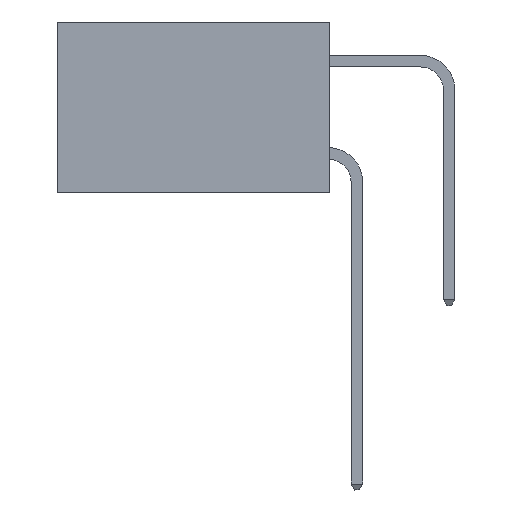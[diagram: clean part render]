
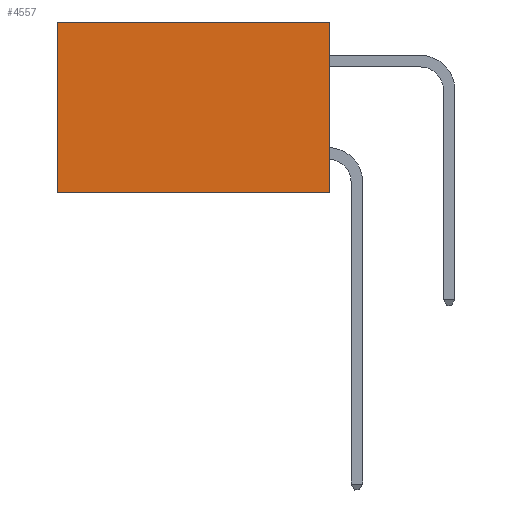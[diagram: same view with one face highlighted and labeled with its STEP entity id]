
A CAD part, left-side view. The second image highlights one B-rep face of the part: STEP entity #4557.
In plain terms, the highlighted planar face has unit normal (-1, 0, 0).
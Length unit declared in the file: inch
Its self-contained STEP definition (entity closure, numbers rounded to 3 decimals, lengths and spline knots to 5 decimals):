
#409 = VECTOR ( 'NONE', #18096, 39.37008 ) ;
#3427 = LINE ( 'NONE', #28919, #17047 ) ;
#3834 = VERTEX_POINT ( 'NONE', #17216 ) ;
#4557 = ADVANCED_FACE ( 'NONE', ( #15839 ), #34240, .F. ) ;
#5149 = ORIENTED_EDGE ( 'NONE', *, *, #21586, .T. ) ;
#5661 = VECTOR ( 'NONE', #33247, 39.37008 ) ;
#6301 = AXIS2_PLACEMENT_3D ( 'NONE', #33501, #33183, #33338 ) ;
#6411 = CARTESIAN_POINT ( 'NONE',  ( 0.277, 0., -0.37 ) ) ;
#6700 = ORIENTED_EDGE ( 'NONE', *, *, #19573, .T. ) ;
#6984 = VERTEX_POINT ( 'NONE', #6411 ) ;
#9887 = DIRECTION ( 'NONE',  ( 0., 1., 0. ) ) ;
#12325 = LINE ( 'NONE', #12391, #25951 ) ;
#12391 = CARTESIAN_POINT ( 'NONE',  ( 0.277, 0.59, -0.37 ) ) ;
#13897 = VERTEX_POINT ( 'NONE', #29089 ) ;
#14819 = ORIENTED_EDGE ( 'NONE', *, *, #19657, .F. ) ;
#15159 = DIRECTION ( 'NONE',  ( 0., 0., -1. ) ) ;
#15195 = VERTEX_POINT ( 'NONE', #26173 ) ;
#15353 = CARTESIAN_POINT ( 'NONE',  ( 0.277, 0., -0.37 ) ) ;
#15839 = FACE_OUTER_BOUND ( 'NONE', #21071, .T. ) ;
#17047 = VECTOR ( 'NONE', #9887, 39.37008 ) ;
#17216 = CARTESIAN_POINT ( 'NONE',  ( 0.277, 0.59, 0. ) ) ;
#18096 = DIRECTION ( 'NONE',  ( 0., 0., -1. ) ) ;
#19573 = EDGE_CURVE ( 'NONE', #3834, #15195, #12325, .T. ) ;
#19657 = EDGE_CURVE ( 'NONE', #6984, #15195, #3427, .T. ) ;
#20057 = ORIENTED_EDGE ( 'NONE', *, *, #30890, .F. ) ;
#21071 = EDGE_LOOP ( 'NONE', ( #6700, #14819, #20057, #5149 ) ) ;
#21586 = EDGE_CURVE ( 'NONE', #13897, #3834, #32765, .T. ) ;
#22113 = LINE ( 'NONE', #15353, #409 ) ;
#25951 = VECTOR ( 'NONE', #15159, 39.37008 ) ;
#26173 = CARTESIAN_POINT ( 'NONE',  ( 0.277, 0.59, -0.37 ) ) ;
#28919 = CARTESIAN_POINT ( 'NONE',  ( 0.277, 0., -0.37 ) ) ;
#29089 = CARTESIAN_POINT ( 'NONE',  ( 0.277, 0., 0. ) ) ;
#30728 = CARTESIAN_POINT ( 'NONE',  ( 0.277, 0., 0. ) ) ;
#30890 = EDGE_CURVE ( 'NONE', #13897, #6984, #22113, .T. ) ;
#32765 = LINE ( 'NONE', #30728, #5661 ) ;
#33183 = DIRECTION ( 'NONE',  ( 1., 0., 0. ) ) ;
#33247 = DIRECTION ( 'NONE',  ( 0., 1., 0. ) ) ;
#33338 = DIRECTION ( 'NONE',  ( 0., 0., -1. ) ) ;
#33501 = CARTESIAN_POINT ( 'NONE',  ( 0.277, 0., -0.37 ) ) ;
#34240 = PLANE ( 'NONE',  #6301 ) ;
